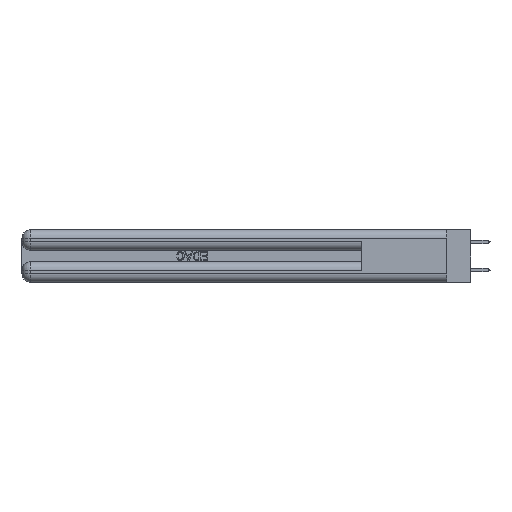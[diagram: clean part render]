
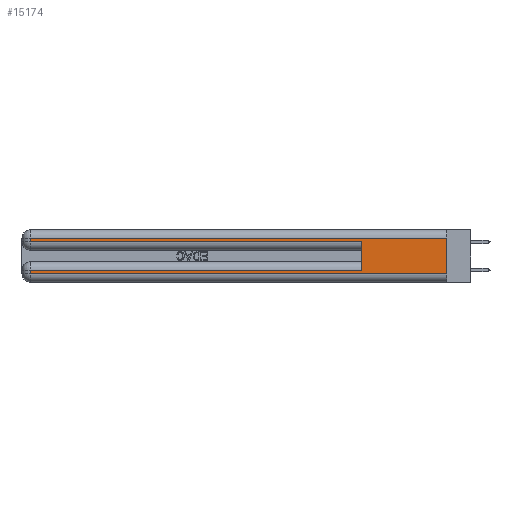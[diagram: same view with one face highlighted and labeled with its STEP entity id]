
A CAD part, left-side view. The second image highlights one B-rep face of the part: STEP entity #15174.
In plain terms, the highlighted planar face has unit normal (-1, 0, 0).
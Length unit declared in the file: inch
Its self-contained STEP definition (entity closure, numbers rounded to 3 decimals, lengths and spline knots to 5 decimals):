
#753 = CARTESIAN_POINT ( 'NONE',  ( 0., 0., 0.085 ) ) ;
#804 = VECTOR ( 'NONE', #11508, 39.37008 ) ;
#1168 = CARTESIAN_POINT ( 'NONE',  ( 0., 2.94, 0.31 ) ) ;
#1763 = VERTEX_POINT ( 'NONE', #9877 ) ;
#1852 = VERTEX_POINT ( 'NONE', #33253 ) ;
#1856 = DIRECTION ( 'NONE',  ( 1., 0., 0. ) ) ;
#2259 = CARTESIAN_POINT ( 'NONE',  ( 0., 0., 0.285 ) ) ;
#2551 = VERTEX_POINT ( 'NONE', #1168 ) ;
#3404 = FACE_OUTER_BOUND ( 'NONE', #40308, .T. ) ;
#3893 = DIRECTION ( 'NONE',  ( 0., 0., -1. ) ) ;
#5304 = PLANE ( 'NONE',  #28158 ) ;
#5444 = VERTEX_POINT ( 'NONE', #44929 ) ;
#5808 = EDGE_CURVE ( 'NONE', #49165, #5444, #34752, .T. ) ;
#6211 = DIRECTION ( 'NONE',  ( 0., -1., 0. ) ) ;
#7288 = VERTEX_POINT ( 'NONE', #43833 ) ;
#7466 = EDGE_CURVE ( 'NONE', #7288, #12175, #19303, .T. ) ;
#7663 = ORIENTED_EDGE ( 'NONE', *, *, #31407, .T. ) ;
#8407 = DIRECTION ( 'NONE',  ( 0., 0., 1. ) ) ;
#9253 = EDGE_CURVE ( 'NONE', #5444, #1852, #13668, .T. ) ;
#9255 = DIRECTION ( 'NONE',  ( 0., 0., -1. ) ) ;
#9301 = LINE ( 'NONE', #18451, #41721 ) ;
#9877 = CARTESIAN_POINT ( 'NONE',  ( 0., 0., 0.31 ) ) ;
#10556 = CARTESIAN_POINT ( 'NONE',  ( 0., 0.6, 0.085 ) ) ;
#11508 = DIRECTION ( 'NONE',  ( 0., -1., 0. ) ) ;
#12175 = VERTEX_POINT ( 'NONE', #20590 ) ;
#13056 = CARTESIAN_POINT ( 'NONE',  ( 0., 2.94, 0.37 ) ) ;
#13631 = VECTOR ( 'NONE', #39898, 39.37008 ) ;
#13668 = LINE ( 'NONE', #23816, #804 ) ;
#14748 = CARTESIAN_POINT ( 'NONE',  ( 0., 2.94, 0.37 ) ) ;
#15174 = ADVANCED_FACE ( 'NONE', ( #3404 ), #5304, .F. ) ;
#15860 = VERTEX_POINT ( 'NONE', #10556 ) ;
#16979 = DIRECTION ( 'NONE',  ( 0., 0., -1. ) ) ;
#17272 = EDGE_CURVE ( 'NONE', #1763, #1852, #9301, .T. ) ;
#17883 = ORIENTED_EDGE ( 'NONE', *, *, #5808, .T. ) ;
#18451 = CARTESIAN_POINT ( 'NONE',  ( 0., 0., 0.37 ) ) ;
#18559 = ORIENTED_EDGE ( 'NONE', *, *, #17272, .F. ) ;
#18695 = EDGE_CURVE ( 'NONE', #15860, #12175, #36353, .T. ) ;
#19303 = LINE ( 'NONE', #2259, #30269 ) ;
#20590 = CARTESIAN_POINT ( 'NONE',  ( 0., 0.6, 0.285 ) ) ;
#20930 = VECTOR ( 'NONE', #16979, 39.37008 ) ;
#21718 = ORIENTED_EDGE ( 'NONE', *, *, #18695, .F. ) ;
#23816 = CARTESIAN_POINT ( 'NONE',  ( 0., 0., 0.06 ) ) ;
#25300 = CARTESIAN_POINT ( 'NONE',  ( 0., 0., 0.37 ) ) ;
#26388 = CARTESIAN_POINT ( 'NONE',  ( 0., 2.94, 0.085 ) ) ;
#26784 = ORIENTED_EDGE ( 'NONE', *, *, #9253, .T. ) ;
#28158 = AXIS2_PLACEMENT_3D ( 'NONE', #25300, #1856, #9255 ) ;
#29369 = EDGE_CURVE ( 'NONE', #2551, #7288, #31329, .T. ) ;
#30269 = VECTOR ( 'NONE', #6211, 39.37008 ) ;
#31329 = LINE ( 'NONE', #13056, #20930 ) ;
#31407 = EDGE_CURVE ( 'NONE', #1763, #2551, #44556, .T. ) ;
#33253 = CARTESIAN_POINT ( 'NONE',  ( 0., 0., 0.06 ) ) ;
#34002 = DIRECTION ( 'NONE',  ( 0., 0., -1. ) ) ;
#34177 = VECTOR ( 'NONE', #34734, 39.37008 ) ;
#34442 = LINE ( 'NONE', #753, #13631 ) ;
#34671 = ORIENTED_EDGE ( 'NONE', *, *, #7466, .T. ) ;
#34734 = DIRECTION ( 'NONE',  ( 0., 1., 0. ) ) ;
#34752 = LINE ( 'NONE', #14748, #47584 ) ;
#35133 = VECTOR ( 'NONE', #8407, 39.37008 ) ;
#35899 = EDGE_CURVE ( 'NONE', #15860, #49165, #34442, .T. ) ;
#36353 = LINE ( 'NONE', #47529, #35133 ) ;
#36884 = ORIENTED_EDGE ( 'NONE', *, *, #29369, .T. ) ;
#39898 = DIRECTION ( 'NONE',  ( 0., 1., 0. ) ) ;
#40308 = EDGE_LOOP ( 'NONE', ( #18559, #7663, #36884, #34671, #21718, #49500, #17883, #26784 ) ) ;
#41721 = VECTOR ( 'NONE', #34002, 39.37008 ) ;
#42598 = CARTESIAN_POINT ( 'NONE',  ( 0., 0., 0.31 ) ) ;
#43833 = CARTESIAN_POINT ( 'NONE',  ( 0., 2.94, 0.285 ) ) ;
#44556 = LINE ( 'NONE', #42598, #34177 ) ;
#44929 = CARTESIAN_POINT ( 'NONE',  ( 0., 2.94, 0.06 ) ) ;
#47529 = CARTESIAN_POINT ( 'NONE',  ( 0., 0.6, 0.145 ) ) ;
#47584 = VECTOR ( 'NONE', #3893, 39.37008 ) ;
#49165 = VERTEX_POINT ( 'NONE', #26388 ) ;
#49500 = ORIENTED_EDGE ( 'NONE', *, *, #35899, .T. ) ;
